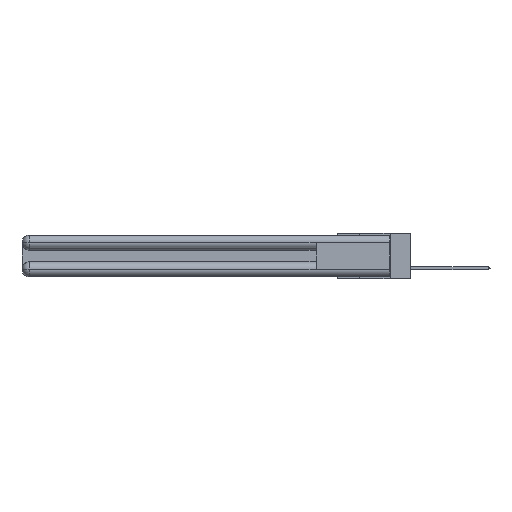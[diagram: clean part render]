
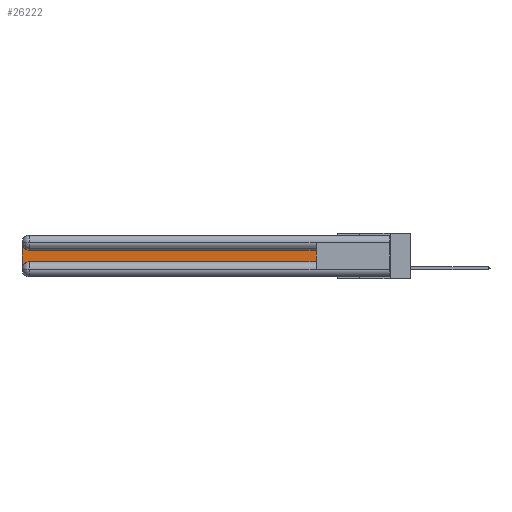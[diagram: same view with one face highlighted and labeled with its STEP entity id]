
A CAD part, left-side view. The second image highlights one B-rep face of the part: STEP entity #26222.
In plain terms, the highlighted planar face has unit normal (-1, 0, 0).
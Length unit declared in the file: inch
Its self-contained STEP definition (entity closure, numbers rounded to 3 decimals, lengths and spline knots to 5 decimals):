
#76 = EDGE_CURVE ( 'NONE', #19048, #17811, #20212, .T. ) ;
#610 = AXIS2_PLACEMENT_3D ( 'NONE', #28467, #13486, #3931 ) ;
#797 = VERTEX_POINT ( 'NONE', #30340 ) ;
#1395 = ORIENTED_EDGE ( 'NONE', *, *, #7138, .T. ) ;
#2118 = ORIENTED_EDGE ( 'NONE', *, *, #28714, .T. ) ;
#2654 = CIRCLE ( 'NONE', #610, 0.06 ) ;
#2757 = CARTESIAN_POINT ( 'NONE',  ( 0.075, 0.6, -0.2175 ) ) ;
#3025 = DIRECTION ( 'NONE',  ( 0., 1., 0. ) ) ;
#3466 = EDGE_CURVE ( 'NONE', #797, #16119, #29297, .T. ) ;
#3931 = DIRECTION ( 'NONE',  ( 0., 0., -1. ) ) ;
#4428 = DIRECTION ( 'NONE',  ( 1., 0., 0. ) ) ;
#4868 = DIRECTION ( 'NONE',  ( 1., 0., 0. ) ) ;
#5834 = ORIENTED_EDGE ( 'NONE', *, *, #16923, .T. ) ;
#6768 = AXIS2_PLACEMENT_3D ( 'NONE', #19754, #4868, #19926 ) ;
#6934 = PLANE ( 'NONE',  #7716 ) ;
#7138 = EDGE_CURVE ( 'NONE', #12103, #797, #31189, .T. ) ;
#7716 = AXIS2_PLACEMENT_3D ( 'NONE', #26695, #4428, #21795 ) ;
#9363 = VECTOR ( 'NONE', #3025, 39.37008 ) ;
#9521 = VECTOR ( 'NONE', #29646, 39.37008 ) ;
#10504 = ORIENTED_EDGE ( 'NONE', *, *, #3466, .T. ) ;
#11764 = DIRECTION ( 'NONE',  ( 0., 0., -1. ) ) ;
#12103 = VERTEX_POINT ( 'NONE', #20496 ) ;
#13150 = CARTESIAN_POINT ( 'NONE',  ( 0.075, 0.6, -0.2175 ) ) ;
#13486 = DIRECTION ( 'NONE',  ( 1., 0., 0. ) ) ;
#15584 = CARTESIAN_POINT ( 'NONE',  ( 0.075, 0.6, -0.1225 ) ) ;
#16089 = LINE ( 'NONE', #22134, #9521 ) ;
#16119 = VERTEX_POINT ( 'NONE', #25672 ) ;
#16923 = EDGE_CURVE ( 'NONE', #20639, #19048, #16089, .T. ) ;
#17811 = VERTEX_POINT ( 'NONE', #19477 ) ;
#18592 = ORIENTED_EDGE ( 'NONE', *, *, #29458, .T. ) ;
#19048 = VERTEX_POINT ( 'NONE', #26103 ) ;
#19477 = CARTESIAN_POINT ( 'NONE',  ( 0.075, 2.94, -0.1225 ) ) ;
#19754 = CARTESIAN_POINT ( 'NONE',  ( 0.075, 2.94, -0.2775 ) ) ;
#19926 = DIRECTION ( 'NONE',  ( 0., 0., -1. ) ) ;
#20120 = DIRECTION ( 'NONE',  ( 0., -1., 0. ) ) ;
#20212 = LINE ( 'NONE', #15584, #9363 ) ;
#20496 = CARTESIAN_POINT ( 'NONE',  ( 0.075, 3., -0.0625 ) ) ;
#20639 = VERTEX_POINT ( 'NONE', #13150 ) ;
#20663 = FACE_OUTER_BOUND ( 'NONE', #31757, .T. ) ;
#20851 = VECTOR ( 'NONE', #20120, 39.37008 ) ;
#21795 = DIRECTION ( 'NONE',  ( 0., 0., -1. ) ) ;
#22134 = CARTESIAN_POINT ( 'NONE',  ( 0.075, 0.6, -0.2175 ) ) ;
#24133 = CARTESIAN_POINT ( 'NONE',  ( 0.075, 3., -0.2175 ) ) ;
#25672 = CARTESIAN_POINT ( 'NONE',  ( 0.075, 2.94, -0.2175 ) ) ;
#26103 = CARTESIAN_POINT ( 'NONE',  ( 0.075, 0.6, -0.1225 ) ) ;
#26222 = ADVANCED_FACE ( 'NONE', ( #20663 ), #6934, .F. ) ;
#26224 = ORIENTED_EDGE ( 'NONE', *, *, #76, .T. ) ;
#26695 = CARTESIAN_POINT ( 'NONE',  ( 0.075, 3., -0.1225 ) ) ;
#28467 = CARTESIAN_POINT ( 'NONE',  ( 0.075, 2.94, -0.0625 ) ) ;
#28597 = LINE ( 'NONE', #2757, #20851 ) ;
#28714 = EDGE_CURVE ( 'NONE', #17811, #12103, #2654, .T. ) ;
#29297 = CIRCLE ( 'NONE', #6768, 0.06 ) ;
#29458 = EDGE_CURVE ( 'NONE', #16119, #20639, #28597, .T. ) ;
#29646 = DIRECTION ( 'NONE',  ( 0., 0., 1. ) ) ;
#30340 = CARTESIAN_POINT ( 'NONE',  ( 0.075, 3., -0.2775 ) ) ;
#31189 = LINE ( 'NONE', #24133, #31945 ) ;
#31757 = EDGE_LOOP ( 'NONE', ( #26224, #2118, #1395, #10504, #18592, #5834 ) ) ;
#31945 = VECTOR ( 'NONE', #11764, 39.37008 ) ;
